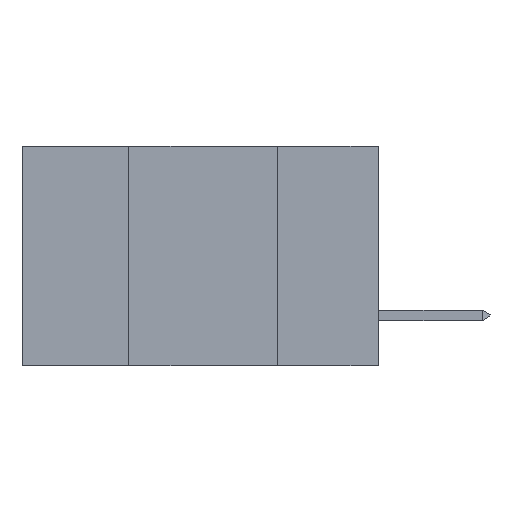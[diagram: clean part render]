
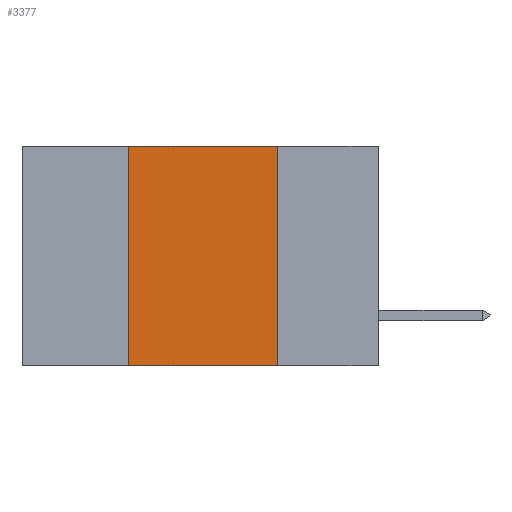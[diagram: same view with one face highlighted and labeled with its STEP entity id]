
A CAD part, left-side view. The second image highlights one B-rep face of the part: STEP entity #3377.
In plain terms, the highlighted planar face has unit normal (-1, 0, 0).
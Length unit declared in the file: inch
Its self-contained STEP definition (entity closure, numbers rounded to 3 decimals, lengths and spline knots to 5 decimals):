
#997 = CARTESIAN_POINT ( 'NONE',  ( 0., 0.6, 0. ) ) ;
#2283 = ORIENTED_EDGE ( 'NONE', *, *, #19103, .F. ) ;
#2961 = VERTEX_POINT ( 'NONE', #22857 ) ;
#3377 = ADVANCED_FACE ( 'NONE', ( #19204 ), #17438, .F. ) ;
#4960 = LINE ( 'NONE', #6811, #15483 ) ;
#4968 = CARTESIAN_POINT ( 'NONE',  ( 0., 0.42, -0.37 ) ) ;
#5936 = CARTESIAN_POINT ( 'NONE',  ( 0., 0.17, -0.37 ) ) ;
#6811 = CARTESIAN_POINT ( 'NONE',  ( 0., 0.17, -0.37 ) ) ;
#8324 = LINE ( 'NONE', #997, #9618 ) ;
#9369 = ORIENTED_EDGE ( 'NONE', *, *, #15396, .F. ) ;
#9618 = VECTOR ( 'NONE', #15433, 39.37008 ) ;
#10219 = CARTESIAN_POINT ( 'NONE',  ( 0., 0.6, 0. ) ) ;
#10768 = DIRECTION ( 'NONE',  ( 0., 0., -1. ) ) ;
#10783 = EDGE_LOOP ( 'NONE', ( #9369, #2283, #17883, #11785 ) ) ;
#11785 = ORIENTED_EDGE ( 'NONE', *, *, #14637, .T. ) ;
#11956 = VERTEX_POINT ( 'NONE', #18314 ) ;
#12027 = DIRECTION ( 'NONE',  ( 0., -1., 0. ) ) ;
#12068 = DIRECTION ( 'NONE',  ( 0., 0., 1. ) ) ;
#13026 = AXIS2_PLACEMENT_3D ( 'NONE', #10219, #20227, #17554 ) ;
#14637 = EDGE_CURVE ( 'NONE', #2961, #16375, #19493, .T. ) ;
#15396 = EDGE_CURVE ( 'NONE', #11956, #16375, #4960, .T. ) ;
#15433 = DIRECTION ( 'NONE',  ( 0., -1., 0. ) ) ;
#15483 = VECTOR ( 'NONE', #10768, 39.37008 ) ;
#16375 = VERTEX_POINT ( 'NONE', #5936 ) ;
#17438 = PLANE ( 'NONE',  #13026 ) ;
#17554 = DIRECTION ( 'NONE',  ( 0., 0., -1. ) ) ;
#17718 = VECTOR ( 'NONE', #12027, 39.37008 ) ;
#17883 = ORIENTED_EDGE ( 'NONE', *, *, #22712, .F. ) ;
#17928 = VECTOR ( 'NONE', #12068, 39.37008 ) ;
#18314 = CARTESIAN_POINT ( 'NONE',  ( 0., 0.17, 0. ) ) ;
#19074 = LINE ( 'NONE', #4968, #17928 ) ;
#19103 = EDGE_CURVE ( 'NONE', #22079, #11956, #8324, .T. ) ;
#19204 = FACE_OUTER_BOUND ( 'NONE', #10783, .T. ) ;
#19493 = LINE ( 'NONE', #21019, #17718 ) ;
#20227 = DIRECTION ( 'NONE',  ( 1., 0., 0. ) ) ;
#21019 = CARTESIAN_POINT ( 'NONE',  ( 0., 0.6, -0.37 ) ) ;
#21138 = CARTESIAN_POINT ( 'NONE',  ( 0., 0.42, 0. ) ) ;
#22079 = VERTEX_POINT ( 'NONE', #21138 ) ;
#22712 = EDGE_CURVE ( 'NONE', #2961, #22079, #19074, .T. ) ;
#22857 = CARTESIAN_POINT ( 'NONE',  ( 0., 0.42, -0.37 ) ) ;
